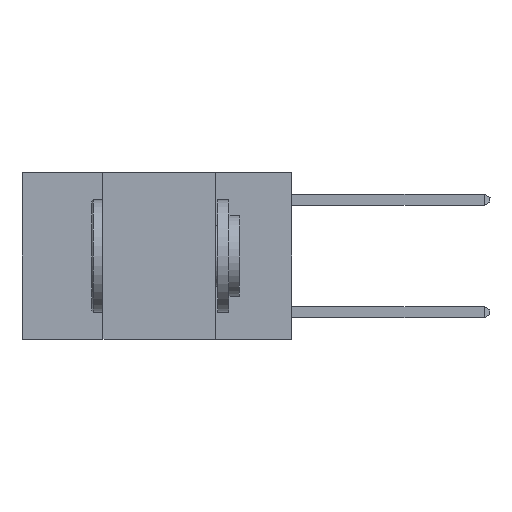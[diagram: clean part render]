
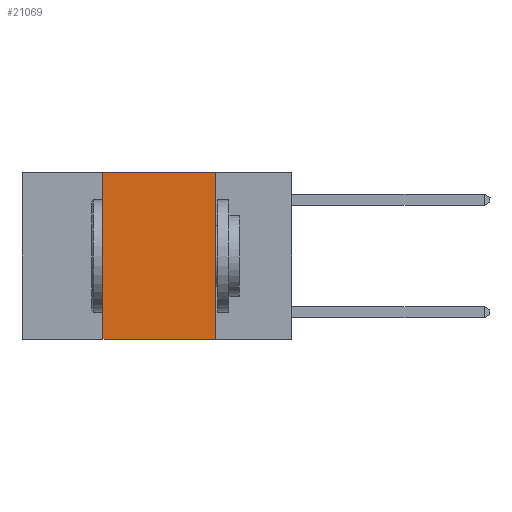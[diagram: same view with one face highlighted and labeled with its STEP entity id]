
A CAD part, left-side view. The second image highlights one B-rep face of the part: STEP entity #21069.
In plain terms, the highlighted planar face has unit normal (-1, 0, 0).
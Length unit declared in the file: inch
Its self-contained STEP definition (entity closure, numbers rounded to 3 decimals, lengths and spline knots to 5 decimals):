
#890 = EDGE_CURVE ( 'NONE', #20046, #18704, #14333, .T. ) ;
#1046 = CARTESIAN_POINT ( 'NONE',  ( 0., 0.42, 0. ) ) ;
#1167 = CARTESIAN_POINT ( 'NONE',  ( 0., 0.6, -0.37 ) ) ;
#2648 = ORIENTED_EDGE ( 'NONE', *, *, #890, .F. ) ;
#2672 = DIRECTION ( 'NONE',  ( 0., -1., 0. ) ) ;
#3351 = DIRECTION ( 'NONE',  ( 0., 0., -1. ) ) ;
#4018 = LINE ( 'NONE', #10545, #11530 ) ;
#4185 = VERTEX_POINT ( 'NONE', #5497 ) ;
#4673 = FACE_OUTER_BOUND ( 'NONE', #5856, .T. ) ;
#5497 = CARTESIAN_POINT ( 'NONE',  ( 0., 0.42, -0.37 ) ) ;
#5640 = CARTESIAN_POINT ( 'NONE',  ( 0., 0.17, -0.37 ) ) ;
#5856 = EDGE_LOOP ( 'NONE', ( #12960, #2648, #20905, #16308 ) ) ;
#6083 = DIRECTION ( 'NONE',  ( 0., -1., 0. ) ) ;
#7026 = DIRECTION ( 'NONE',  ( 0., 0., -1. ) ) ;
#7707 = LINE ( 'NONE', #1167, #12426 ) ;
#7963 = VERTEX_POINT ( 'NONE', #5640 ) ;
#8049 = CARTESIAN_POINT ( 'NONE',  ( 0., 0.6, 0. ) ) ;
#8079 = VECTOR ( 'NONE', #7026, 39.37008 ) ;
#10545 = CARTESIAN_POINT ( 'NONE',  ( 0., 0.42, 0. ) ) ;
#11530 = VECTOR ( 'NONE', #17017, 39.37008 ) ;
#11569 = CARTESIAN_POINT ( 'NONE',  ( 0., 0.17, 0. ) ) ;
#12081 = VECTOR ( 'NONE', #6083, 39.37008 ) ;
#12426 = VECTOR ( 'NONE', #2672, 39.37008 ) ;
#12960 = ORIENTED_EDGE ( 'NONE', *, *, #18514, .F. ) ;
#13166 = EDGE_CURVE ( 'NONE', #4185, #7963, #7707, .T. ) ;
#14333 = LINE ( 'NONE', #20906, #12081 ) ;
#14644 = AXIS2_PLACEMENT_3D ( 'NONE', #8049, #19608, #3351 ) ;
#15262 = LINE ( 'NONE', #16663, #8079 ) ;
#16308 = ORIENTED_EDGE ( 'NONE', *, *, #13166, .T. ) ;
#16663 = CARTESIAN_POINT ( 'NONE',  ( 0., 0.17, 0. ) ) ;
#17017 = DIRECTION ( 'NONE',  ( 0., 0., 1. ) ) ;
#18099 = PLANE ( 'NONE',  #14644 ) ;
#18514 = EDGE_CURVE ( 'NONE', #18704, #7963, #15262, .T. ) ;
#18704 = VERTEX_POINT ( 'NONE', #11569 ) ;
#19608 = DIRECTION ( 'NONE',  ( 1., 0., 0. ) ) ;
#20046 = VERTEX_POINT ( 'NONE', #1046 ) ;
#20708 = EDGE_CURVE ( 'NONE', #4185, #20046, #4018, .T. ) ;
#20905 = ORIENTED_EDGE ( 'NONE', *, *, #20708, .F. ) ;
#20906 = CARTESIAN_POINT ( 'NONE',  ( 0., 0.6, 0. ) ) ;
#21069 = ADVANCED_FACE ( 'NONE', ( #4673 ), #18099, .F. ) ;
